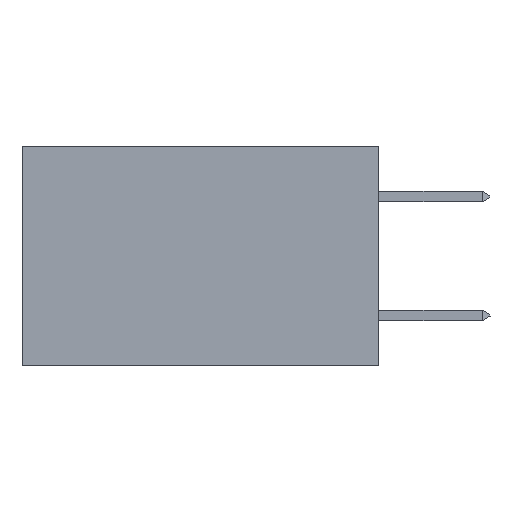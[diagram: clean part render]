
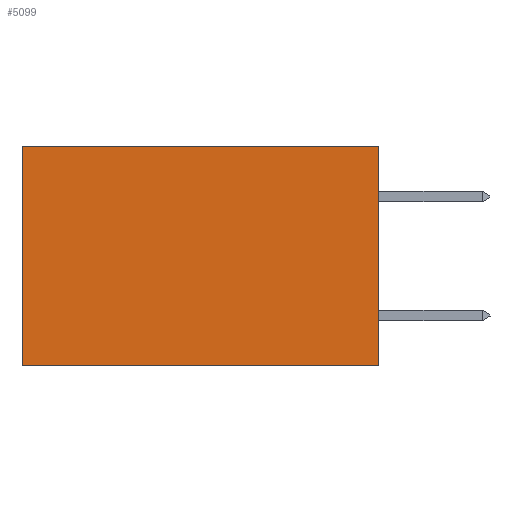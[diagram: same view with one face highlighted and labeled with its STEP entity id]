
A CAD part, left-side view. The second image highlights one B-rep face of the part: STEP entity #5099.
In plain terms, the highlighted planar face has unit normal (-1, 0, 0).
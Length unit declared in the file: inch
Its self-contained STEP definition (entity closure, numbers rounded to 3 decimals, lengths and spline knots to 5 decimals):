
#1156 = ORIENTED_EDGE ( 'NONE', *, *, #6145, .T. ) ;
#1791 = LINE ( 'NONE', #3735, #21476 ) ;
#2508 = VECTOR ( 'NONE', #17970, 39.37008 ) ;
#2690 = CARTESIAN_POINT ( 'NONE',  ( 0.298, 0., 0. ) ) ;
#3627 = VERTEX_POINT ( 'NONE', #8710 ) ;
#3735 = CARTESIAN_POINT ( 'NONE',  ( 0.298, 0.6, 0. ) ) ;
#4341 = DIRECTION ( 'NONE',  ( 0., 1., 0. ) ) ;
#4749 = CARTESIAN_POINT ( 'NONE',  ( 0.298, 0., 0. ) ) ;
#5099 = ADVANCED_FACE ( 'NONE', ( #18119 ), #18608, .F. ) ;
#5139 = LINE ( 'NONE', #23582, #19759 ) ;
#5609 = DIRECTION ( 'NONE',  ( 0., 0., -1. ) ) ;
#5753 = EDGE_LOOP ( 'NONE', ( #19852, #12269, #8843, #1156 ) ) ;
#6145 = EDGE_CURVE ( 'NONE', #14487, #6669, #23312, .T. ) ;
#6669 = VERTEX_POINT ( 'NONE', #14773 ) ;
#7523 = VECTOR ( 'NONE', #4341, 39.37008 ) ;
#7840 = CARTESIAN_POINT ( 'NONE',  ( 0.298, 0.6, -0.37 ) ) ;
#8710 = CARTESIAN_POINT ( 'NONE',  ( 0.298, 0., -0.37 ) ) ;
#8843 = ORIENTED_EDGE ( 'NONE', *, *, #8874, .F. ) ;
#8874 = EDGE_CURVE ( 'NONE', #14487, #3627, #16547, .T. ) ;
#10325 = DIRECTION ( 'NONE',  ( 1., 0., 0. ) ) ;
#12269 = ORIENTED_EDGE ( 'NONE', *, *, #15519, .F. ) ;
#13790 = AXIS2_PLACEMENT_3D ( 'NONE', #23807, #10325, #23847 ) ;
#14191 = DIRECTION ( 'NONE',  ( 0., 1., 0. ) ) ;
#14487 = VERTEX_POINT ( 'NONE', #24107 ) ;
#14773 = CARTESIAN_POINT ( 'NONE',  ( 0.298, 0.6, 0. ) ) ;
#15519 = EDGE_CURVE ( 'NONE', #3627, #16025, #5139, .T. ) ;
#16025 = VERTEX_POINT ( 'NONE', #7840 ) ;
#16547 = LINE ( 'NONE', #2690, #2508 ) ;
#16812 = EDGE_CURVE ( 'NONE', #6669, #16025, #1791, .T. ) ;
#17970 = DIRECTION ( 'NONE',  ( 0., 0., -1. ) ) ;
#18119 = FACE_OUTER_BOUND ( 'NONE', #5753, .T. ) ;
#18608 = PLANE ( 'NONE',  #13790 ) ;
#19759 = VECTOR ( 'NONE', #14191, 39.37008 ) ;
#19852 = ORIENTED_EDGE ( 'NONE', *, *, #16812, .T. ) ;
#21476 = VECTOR ( 'NONE', #5609, 39.37008 ) ;
#23312 = LINE ( 'NONE', #4749, #7523 ) ;
#23582 = CARTESIAN_POINT ( 'NONE',  ( 0.298, 0., -0.37 ) ) ;
#23807 = CARTESIAN_POINT ( 'NONE',  ( 0.298, 0., 0. ) ) ;
#23847 = DIRECTION ( 'NONE',  ( 0., 0., -1. ) ) ;
#24107 = CARTESIAN_POINT ( 'NONE',  ( 0.298, 0., 0. ) ) ;
